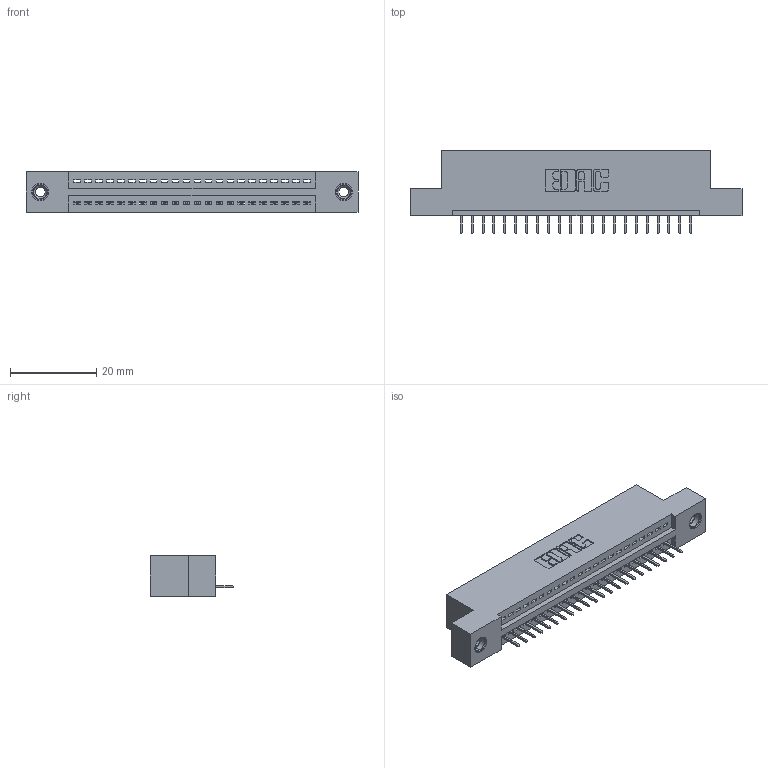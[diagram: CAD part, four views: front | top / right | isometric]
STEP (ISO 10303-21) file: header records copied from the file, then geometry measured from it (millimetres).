
FILE_DESCRIPTION (( 'STEP AP203' ), '1' );
FILE_NAME ('345-022-524-108.STEP', '2019-10-05T00:07:17', ( '' ), ( '' ), 'SwSTEP 2.0', 'SolidWorks 2016', '' );
FILE_SCHEMA (( 'CONFIG_CONTROL_DESIGN' ));
Length unit declared in the file: inch
Products named in the file (4): 345-292-001_345-293-124; 345-250-001_345-250-003-102; 345 Part_Flush Mounting Lugs - 0.156 Dia-TI; 345-022-524-108
Assembly tree (25 placements, depth 2):
  345-022-524-108
    345 Part_Flush Mounting Lugs - 0.156 Dia-TI
    345-292-001_345-293-124  x22
    345-250-001_345-250-003-102  x2
Bounding box: 77.09 x 19.35 x 9.4 mm (x, y, z)
Volume: 7064.7 mm3; surface area: 8857.9 mm2
Topology: 25 solids, 25 shells, 1550 faces, 4437 edges, 2862 vertices
Faces by surface type: plane 1124, cylinder 410, cone 12, torus 4
Entity records: 20510 total; most frequent: CARTESIAN_POINT 3533, ORIENTED_EDGE 3482, DIRECTION 3143, EDGE_CURVE 1741, LINE 1505, VECTOR 1505, VERTEX_POINT 1152, AXIS2_PLACEMENT_3D 819
